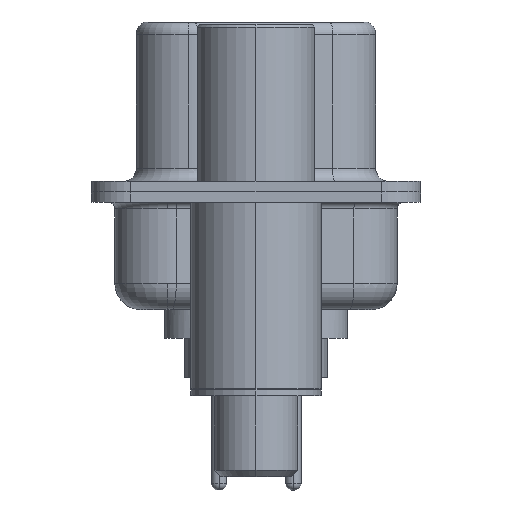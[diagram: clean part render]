
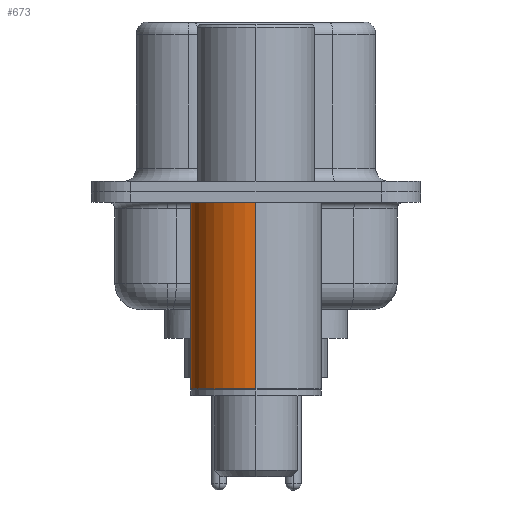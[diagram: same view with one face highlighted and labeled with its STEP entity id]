
A CAD part, left-side view. The second image highlights one B-rep face of the part: STEP entity #673.
In plain terms, the highlighted cylindrical face has radius 2.5 mm (diameter 5 mm), a partial arc.
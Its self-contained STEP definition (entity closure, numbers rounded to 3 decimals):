
#325 = ORIENTED_EDGE ( 'NONE', *, *, #2568, .F. ) ;
#659 = ORIENTED_EDGE ( 'NONE', *, *, #9072, .F. ) ;
#673 = ADVANCED_FACE ( 'NONE', ( #14107 ), #6602, .T. ) ;
#983 = CARTESIAN_POINT ( 'NONE',  ( 0., 0., 0.581 ) ) ;
#1246 = EDGE_CURVE ( 'NONE', #9442, #13295, #2274, .T. ) ;
#1456 = ORIENTED_EDGE ( 'NONE', *, *, #1246, .T. ) ;
#2274 = CIRCLE ( 'NONE', #4626, 2.5 ) ;
#2568 = EDGE_CURVE ( 'NONE', #4875, #8080, #8907, .T. ) ;
#2931 = CARTESIAN_POINT ( 'NONE',  ( 2.5, 0., -7.525 ) ) ;
#2956 = CARTESIAN_POINT ( 'NONE',  ( 2.5, 0., 0.581 ) ) ;
#4285 = AXIS2_PLACEMENT_3D ( 'NONE', #983, #14254, #19141 ) ;
#4626 = AXIS2_PLACEMENT_3D ( 'NONE', #9393, #14231, #6074 ) ;
#4875 = VERTEX_POINT ( 'NONE', #15238 ) ;
#5348 = VECTOR ( 'NONE', #6158, 1000. ) ;
#5793 = VECTOR ( 'NONE', #19430, 1000. ) ;
#6074 = DIRECTION ( 'NONE',  ( 1., 0., 0. ) ) ;
#6158 = DIRECTION ( 'NONE',  ( 0., 0., 1. ) ) ;
#6602 = CYLINDRICAL_SURFACE ( 'NONE', #4285, 2.5 ) ;
#8080 = VERTEX_POINT ( 'NONE', #15700 ) ;
#8346 = LINE ( 'NONE', #2956, #5793 ) ;
#8907 = CIRCLE ( 'NONE', #16662, 2.5 ) ;
#9072 = EDGE_CURVE ( 'NONE', #9442, #4875, #8346, .T. ) ;
#9393 = CARTESIAN_POINT ( 'NONE',  ( 0., 0., -7.525 ) ) ;
#9442 = VERTEX_POINT ( 'NONE', #2931 ) ;
#10040 = ORIENTED_EDGE ( 'NONE', *, *, #18506, .T. ) ;
#11000 = CARTESIAN_POINT ( 'NONE',  ( 0., 0., -0.4 ) ) ;
#12387 = CARTESIAN_POINT ( 'NONE',  ( -2.5, 0., -7.525 ) ) ;
#13295 = VERTEX_POINT ( 'NONE', #12387 ) ;
#14107 = FACE_OUTER_BOUND ( 'NONE', #18187, .T. ) ;
#14231 = DIRECTION ( 'NONE',  ( 0., 0., 1. ) ) ;
#14254 = DIRECTION ( 'NONE',  ( 0., 0., 1. ) ) ;
#14376 = CARTESIAN_POINT ( 'NONE',  ( -2.5, 0., 0.581 ) ) ;
#15238 = CARTESIAN_POINT ( 'NONE',  ( 2.5, 0., -0.4 ) ) ;
#15700 = CARTESIAN_POINT ( 'NONE',  ( -2.5, 0., -0.4 ) ) ;
#16045 = DIRECTION ( 'NONE',  ( 0., 0., 1. ) ) ;
#16662 = AXIS2_PLACEMENT_3D ( 'NONE', #11000, #16045, #17690 ) ;
#17690 = DIRECTION ( 'NONE',  ( 1., 0., 0. ) ) ;
#18187 = EDGE_LOOP ( 'NONE', ( #1456, #10040, #325, #659 ) ) ;
#18506 = EDGE_CURVE ( 'NONE', #13295, #8080, #21056, .T. ) ;
#19141 = DIRECTION ( 'NONE',  ( 1., 0., 0. ) ) ;
#19430 = DIRECTION ( 'NONE',  ( 0., 0., 1. ) ) ;
#21056 = LINE ( 'NONE', #14376, #5348 ) ;
